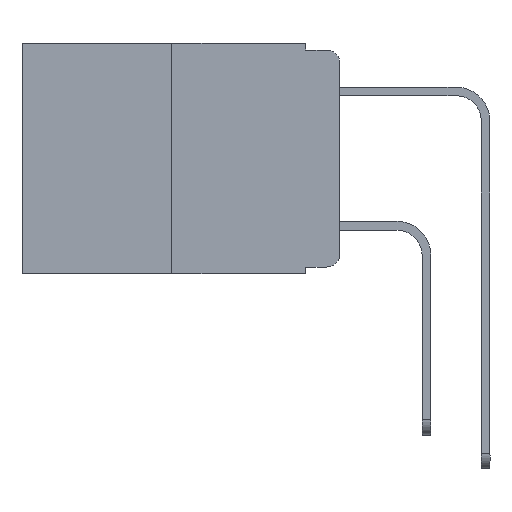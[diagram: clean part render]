
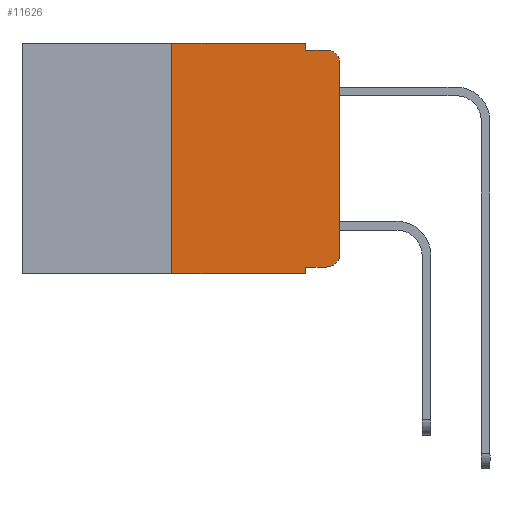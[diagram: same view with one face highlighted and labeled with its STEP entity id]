
A CAD part, left-side view. The second image highlights one B-rep face of the part: STEP entity #11626.
In plain terms, the highlighted planar face has unit normal (-1, 0, 0).
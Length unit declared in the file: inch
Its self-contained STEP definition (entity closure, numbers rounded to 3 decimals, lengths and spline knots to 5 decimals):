
#238 = VERTEX_POINT ( 'NONE', #10287 ) ;
#252 = AXIS2_PLACEMENT_3D ( 'NONE', #4446, #8310, #7729 ) ;
#310 = ORIENTED_EDGE ( 'NONE', *, *, #9161, .F. ) ;
#378 = EDGE_CURVE ( 'NONE', #6258, #787, #5647, .T. ) ;
#395 = CARTESIAN_POINT ( 'NONE',  ( 0., 0.25, -0.343 ) ) ;
#493 = VECTOR ( 'NONE', #1963, 39.37008 ) ;
#629 = VERTEX_POINT ( 'NONE', #3115 ) ;
#736 = EDGE_LOOP ( 'NONE', ( #9316, #6940, #6220, #6576, #4012, #310, #5049, #11936, #5465, #1716 ) ) ;
#787 = VERTEX_POINT ( 'NONE', #12204 ) ;
#932 = DIRECTION ( 'NONE',  ( 0., 0., 1. ) ) ;
#994 = VECTOR ( 'NONE', #10975, 39.37008 ) ;
#1240 = EDGE_CURVE ( 'NONE', #3741, #10195, #11364, .T. ) ;
#1338 = LINE ( 'NONE', #5027, #10451 ) ;
#1349 = CARTESIAN_POINT ( 'NONE',  ( 0., 0.02, -0.333 ) ) ;
#1716 = ORIENTED_EDGE ( 'NONE', *, *, #378, .T. ) ;
#1963 = DIRECTION ( 'NONE',  ( 0., 0., -1. ) ) ;
#2143 = CARTESIAN_POINT ( 'NONE',  ( 0., 0.051, 0. ) ) ;
#2149 = CARTESIAN_POINT ( 'NONE',  ( 0., 0.473, -0.343 ) ) ;
#2211 = EDGE_CURVE ( 'NONE', #787, #3741, #11537, .T. ) ;
#2535 = EDGE_CURVE ( 'NONE', #4725, #6258, #8283, .T. ) ;
#2663 = CARTESIAN_POINT ( 'NONE',  ( 0., 0.051, -0.333 ) ) ;
#2906 = AXIS2_PLACEMENT_3D ( 'NONE', #6809, #11760, #7758 ) ;
#2980 = CARTESIAN_POINT ( 'NONE',  ( 0., 0.473, 0. ) ) ;
#3098 = VECTOR ( 'NONE', #11772, 39.37008 ) ;
#3115 = CARTESIAN_POINT ( 'NONE',  ( 0., 0.051, -0.01 ) ) ;
#3139 = VECTOR ( 'NONE', #4693, 39.37008 ) ;
#3542 = CARTESIAN_POINT ( 'NONE',  ( 0., 0.02, -0.01 ) ) ;
#3605 = VECTOR ( 'NONE', #11800, 39.37008 ) ;
#3741 = VERTEX_POINT ( 'NONE', #10350 ) ;
#3850 = EDGE_CURVE ( 'NONE', #4725, #4321, #8734, .T. ) ;
#3989 = PLANE ( 'NONE',  #2906 ) ;
#4012 = ORIENTED_EDGE ( 'NONE', *, *, #11183, .F. ) ;
#4024 = LINE ( 'NONE', #8679, #3605 ) ;
#4275 = DIRECTION ( 'NONE',  ( 0., -1., 0. ) ) ;
#4321 = VERTEX_POINT ( 'NONE', #6706 ) ;
#4446 = CARTESIAN_POINT ( 'NONE',  ( 0., 0.02, -0.313 ) ) ;
#4693 = DIRECTION ( 'NONE',  ( 0., 0., -1. ) ) ;
#4725 = VERTEX_POINT ( 'NONE', #9670 ) ;
#5027 = CARTESIAN_POINT ( 'NONE',  ( 0., 0.051, -0.01 ) ) ;
#5049 = ORIENTED_EDGE ( 'NONE', *, *, #7031, .T. ) ;
#5465 = ORIENTED_EDGE ( 'NONE', *, *, #2535, .T. ) ;
#5537 = DIRECTION ( 'NONE',  ( 0., 0., -1. ) ) ;
#5647 = CIRCLE ( 'NONE', #252, 0.02 ) ;
#6220 = ORIENTED_EDGE ( 'NONE', *, *, #6564, .F. ) ;
#6258 = VERTEX_POINT ( 'NONE', #1349 ) ;
#6318 = DIRECTION ( 'NONE',  ( 0., -1., 0. ) ) ;
#6421 = CARTESIAN_POINT ( 'NONE',  ( 0., 0.02, -0.03 ) ) ;
#6564 = EDGE_CURVE ( 'NONE', #629, #10195, #1338, .T. ) ;
#6576 = ORIENTED_EDGE ( 'NONE', *, *, #7412, .F. ) ;
#6706 = CARTESIAN_POINT ( 'NONE',  ( 0., 0.051, -0.343 ) ) ;
#6809 = CARTESIAN_POINT ( 'NONE',  ( 0., 0.473, 0. ) ) ;
#6940 = ORIENTED_EDGE ( 'NONE', *, *, #1240, .T. ) ;
#7016 = VERTEX_POINT ( 'NONE', #8118 ) ;
#7031 = EDGE_CURVE ( 'NONE', #7698, #4321, #9118, .T. ) ;
#7412 = EDGE_CURVE ( 'NONE', #7016, #629, #9631, .T. ) ;
#7444 = DIRECTION ( 'NONE',  ( -1., 0., 0. ) ) ;
#7698 = VERTEX_POINT ( 'NONE', #395 ) ;
#7729 = DIRECTION ( 'NONE',  ( 0., 0., -1. ) ) ;
#7758 = DIRECTION ( 'NONE',  ( 0., 0., -1. ) ) ;
#8118 = CARTESIAN_POINT ( 'NONE',  ( 0., 0.051, 0. ) ) ;
#8283 = LINE ( 'NONE', #2663, #11746 ) ;
#8310 = DIRECTION ( 'NONE',  ( -1., 0., 0. ) ) ;
#8679 = CARTESIAN_POINT ( 'NONE',  ( 0., 0.25, 0. ) ) ;
#8734 = LINE ( 'NONE', #2143, #493 ) ;
#9118 = LINE ( 'NONE', #2149, #994 ) ;
#9161 = EDGE_CURVE ( 'NONE', #7698, #238, #4024, .T. ) ;
#9316 = ORIENTED_EDGE ( 'NONE', *, *, #2211, .T. ) ;
#9631 = LINE ( 'NONE', #11485, #3139 ) ;
#9670 = CARTESIAN_POINT ( 'NONE',  ( 0., 0.051, -0.333 ) ) ;
#9753 = CARTESIAN_POINT ( 'NONE',  ( 0., 0., 0. ) ) ;
#10195 = VERTEX_POINT ( 'NONE', #3542 ) ;
#10287 = CARTESIAN_POINT ( 'NONE',  ( 0., 0.25, 0. ) ) ;
#10350 = CARTESIAN_POINT ( 'NONE',  ( 0., 0., -0.03 ) ) ;
#10451 = VECTOR ( 'NONE', #4275, 39.37008 ) ;
#10557 = FACE_OUTER_BOUND ( 'NONE', #736, .T. ) ;
#10757 = LINE ( 'NONE', #2980, #3098 ) ;
#10937 = VECTOR ( 'NONE', #932, 39.37008 ) ;
#10975 = DIRECTION ( 'NONE',  ( 0., -1., 0. ) ) ;
#11183 = EDGE_CURVE ( 'NONE', #238, #7016, #10757, .T. ) ;
#11364 = CIRCLE ( 'NONE', #11951, 0.02 ) ;
#11485 = CARTESIAN_POINT ( 'NONE',  ( 0., 0.051, 0. ) ) ;
#11537 = LINE ( 'NONE', #9753, #10937 ) ;
#11626 = ADVANCED_FACE ( 'NONE', ( #10557 ), #3989, .F. ) ;
#11746 = VECTOR ( 'NONE', #6318, 39.37008 ) ;
#11760 = DIRECTION ( 'NONE',  ( 1., 0., 0. ) ) ;
#11772 = DIRECTION ( 'NONE',  ( 0., -1., 0. ) ) ;
#11800 = DIRECTION ( 'NONE',  ( 0., 0., 1. ) ) ;
#11936 = ORIENTED_EDGE ( 'NONE', *, *, #3850, .F. ) ;
#11951 = AXIS2_PLACEMENT_3D ( 'NONE', #6421, #7444, #5537 ) ;
#12204 = CARTESIAN_POINT ( 'NONE',  ( 0., 0., -0.313 ) ) ;
